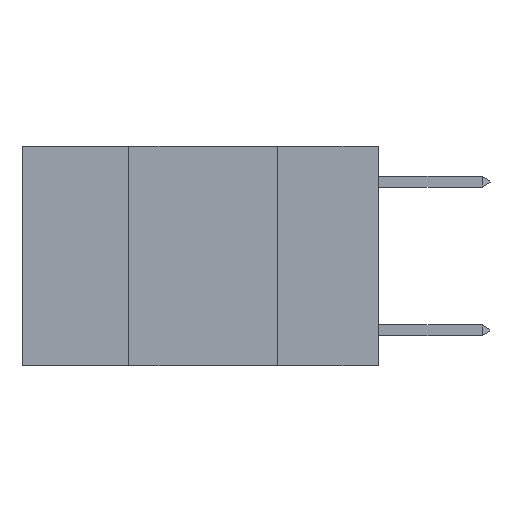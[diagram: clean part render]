
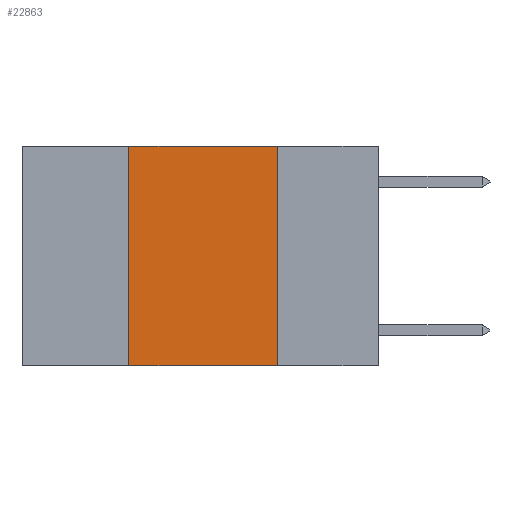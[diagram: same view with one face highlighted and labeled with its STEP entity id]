
A CAD part, left-side view. The second image highlights one B-rep face of the part: STEP entity #22863.
In plain terms, the highlighted planar face has unit normal (-1, 0, 0).
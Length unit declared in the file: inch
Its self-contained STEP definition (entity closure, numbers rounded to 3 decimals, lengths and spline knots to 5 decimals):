
#938 = VECTOR ( 'NONE', #10546, 39.37008 ) ;
#1270 = CARTESIAN_POINT ( 'NONE',  ( 0., 0.17, 0. ) ) ;
#1379 = DIRECTION ( 'NONE',  ( 0., 0., -1. ) ) ;
#1520 = EDGE_CURVE ( 'NONE', #28124, #18300, #17334, .T. ) ;
#1545 = VECTOR ( 'NONE', #22361, 39.37008 ) ;
#1922 = EDGE_CURVE ( 'NONE', #9877, #18300, #25756, .T. ) ;
#4486 = CARTESIAN_POINT ( 'NONE',  ( 0., 0.6, -0.37 ) ) ;
#7793 = LINE ( 'NONE', #21571, #938 ) ;
#7962 = EDGE_CURVE ( 'NONE', #9877, #21068, #7793, .T. ) ;
#8251 = DIRECTION ( 'NONE',  ( 1., 0., 0. ) ) ;
#9701 = CARTESIAN_POINT ( 'NONE',  ( 0., 0.17, -0.37 ) ) ;
#9877 = VERTEX_POINT ( 'NONE', #29037 ) ;
#10546 = DIRECTION ( 'NONE',  ( 0., 0., 1. ) ) ;
#11259 = EDGE_LOOP ( 'NONE', ( #28955, #27937, #23463, #11874 ) ) ;
#11565 = AXIS2_PLACEMENT_3D ( 'NONE', #22321, #8251, #1379 ) ;
#11874 = ORIENTED_EDGE ( 'NONE', *, *, #1922, .T. ) ;
#14305 = DIRECTION ( 'NONE',  ( 0., -1., 0. ) ) ;
#16445 = LINE ( 'NONE', #21489, #17235 ) ;
#17235 = VECTOR ( 'NONE', #14305, 39.37008 ) ;
#17334 = LINE ( 'NONE', #1270, #1545 ) ;
#18300 = VERTEX_POINT ( 'NONE', #9701 ) ;
#21068 = VERTEX_POINT ( 'NONE', #29691 ) ;
#21489 = CARTESIAN_POINT ( 'NONE',  ( 0., 0.6, 0. ) ) ;
#21571 = CARTESIAN_POINT ( 'NONE',  ( 0., 0.42, 0. ) ) ;
#22061 = VECTOR ( 'NONE', #23598, 39.37008 ) ;
#22321 = CARTESIAN_POINT ( 'NONE',  ( 0., 0.6, 0. ) ) ;
#22361 = DIRECTION ( 'NONE',  ( 0., 0., -1. ) ) ;
#22630 = FACE_OUTER_BOUND ( 'NONE', #11259, .T. ) ;
#22863 = ADVANCED_FACE ( 'NONE', ( #22630 ), #26784, .F. ) ;
#23463 = ORIENTED_EDGE ( 'NONE', *, *, #7962, .F. ) ;
#23598 = DIRECTION ( 'NONE',  ( 0., -1., 0. ) ) ;
#25756 = LINE ( 'NONE', #4486, #22061 ) ;
#26198 = CARTESIAN_POINT ( 'NONE',  ( 0., 0.17, 0. ) ) ;
#26784 = PLANE ( 'NONE',  #11565 ) ;
#27937 = ORIENTED_EDGE ( 'NONE', *, *, #29307, .F. ) ;
#28124 = VERTEX_POINT ( 'NONE', #26198 ) ;
#28955 = ORIENTED_EDGE ( 'NONE', *, *, #1520, .F. ) ;
#29037 = CARTESIAN_POINT ( 'NONE',  ( 0., 0.42, -0.37 ) ) ;
#29307 = EDGE_CURVE ( 'NONE', #21068, #28124, #16445, .T. ) ;
#29691 = CARTESIAN_POINT ( 'NONE',  ( 0., 0.42, 0. ) ) ;
